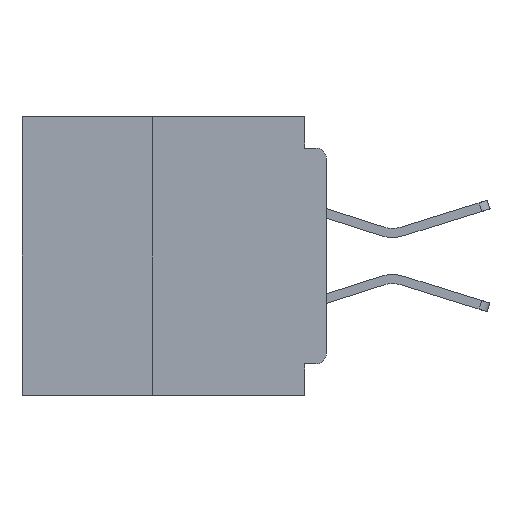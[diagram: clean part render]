
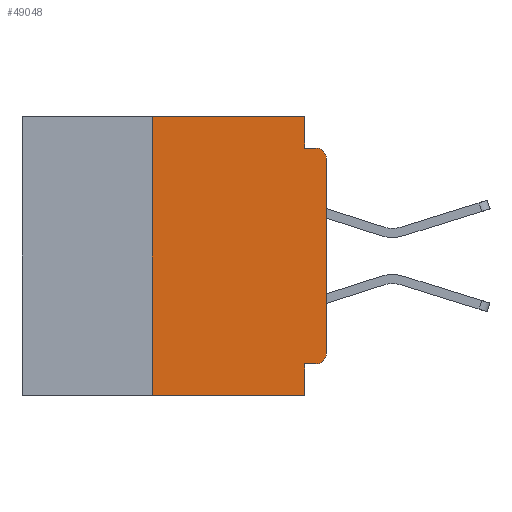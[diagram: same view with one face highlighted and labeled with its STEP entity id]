
A CAD part, left-side view. The second image highlights one B-rep face of the part: STEP entity #49048.
In plain terms, the highlighted planar face has unit normal (-1, 0, 0).
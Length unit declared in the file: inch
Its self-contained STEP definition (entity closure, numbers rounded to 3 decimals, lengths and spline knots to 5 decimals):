
#20 = LINE ( 'NONE', #26239, #21455 ) ;
#35 = EDGE_CURVE ( 'NONE', #26544, #19122, #11716, .T. ) ;
#307 = VECTOR ( 'NONE', #14128, 39.37008 ) ;
#1323 = ORIENTED_EDGE ( 'NONE', *, *, #14427, .F. ) ;
#2789 = CARTESIAN_POINT ( 'NONE',  ( 0., 0., -0.045 ) ) ;
#2907 = EDGE_CURVE ( 'NONE', #47723, #47539, #22066, .T. ) ;
#3143 = DIRECTION ( 'NONE',  ( -1., 0., 0. ) ) ;
#3604 = DIRECTION ( 'NONE',  ( 0., 0., -1. ) ) ;
#3890 = DIRECTION ( 'NONE',  ( 0., 0., -1. ) ) ;
#4039 = VERTEX_POINT ( 'NONE', #25247 ) ;
#4975 = LINE ( 'NONE', #16360, #26354 ) ;
#5308 = ORIENTED_EDGE ( 'NONE', *, *, #29322, .F. ) ;
#5551 = CARTESIAN_POINT ( 'NONE',  ( 0., 0., -0.355 ) ) ;
#8605 = AXIS2_PLACEMENT_3D ( 'NONE', #28709, #3143, #33030 ) ;
#9223 = LINE ( 'NONE', #5551, #20586 ) ;
#9282 = DIRECTION ( 'NONE',  ( 0., 0., 1. ) ) ;
#9868 = DIRECTION ( 'NONE',  ( 0., 1., 0. ) ) ;
#10006 = ORIENTED_EDGE ( 'NONE', *, *, #25366, .T. ) ;
#10900 = CARTESIAN_POINT ( 'NONE',  ( 0., 0.031, 0. ) ) ;
#11251 = FACE_OUTER_BOUND ( 'NONE', #22748, .T. ) ;
#11534 = EDGE_CURVE ( 'NONE', #47723, #33958, #36647, .T. ) ;
#11557 = ORIENTED_EDGE ( 'NONE', *, *, #49314, .F. ) ;
#11716 = LINE ( 'NONE', #20911, #307 ) ;
#12443 = VERTEX_POINT ( 'NONE', #46389 ) ;
#13977 = VECTOR ( 'NONE', #43879, 39.37008 ) ;
#14128 = DIRECTION ( 'NONE',  ( 0., 0., -1. ) ) ;
#14427 = EDGE_CURVE ( 'NONE', #39113, #33958, #4975, .T. ) ;
#14734 = CARTESIAN_POINT ( 'NONE',  ( 0., 0.031, -0.045 ) ) ;
#16360 = CARTESIAN_POINT ( 'NONE',  ( 0., 0.031, -0.4 ) ) ;
#16867 = EDGE_CURVE ( 'NONE', #4039, #47789, #35432, .T. ) ;
#17619 = DIRECTION ( 'NONE',  ( 0., -1., 0. ) ) ;
#19122 = VERTEX_POINT ( 'NONE', #14734 ) ;
#19386 = VECTOR ( 'NONE', #49608, 39.37008 ) ;
#19668 = ORIENTED_EDGE ( 'NONE', *, *, #11534, .T. ) ;
#20367 = ORIENTED_EDGE ( 'NONE', *, *, #16867, .T. ) ;
#20586 = VECTOR ( 'NONE', #9868, 39.37008 ) ;
#20911 = CARTESIAN_POINT ( 'NONE',  ( 0., 0.031, 0. ) ) ;
#20925 = DIRECTION ( 'NONE',  ( -1., 0., 0. ) ) ;
#21347 = CARTESIAN_POINT ( 'NONE',  ( 0., 0.25, 0. ) ) ;
#21455 = VECTOR ( 'NONE', #9282, 39.37008 ) ;
#22066 = LINE ( 'NONE', #30630, #43384 ) ;
#22748 = EDGE_LOOP ( 'NONE', ( #41684, #20367, #5308, #37859, #40615, #23875, #19668, #1323, #11557, #10006 ) ) ;
#23367 = VECTOR ( 'NONE', #17619, 39.37008 ) ;
#23875 = ORIENTED_EDGE ( 'NONE', *, *, #2907, .F. ) ;
#25156 = PLANE ( 'NONE',  #40611 ) ;
#25247 = CARTESIAN_POINT ( 'NONE',  ( 0., 0., -0.06 ) ) ;
#25366 = EDGE_CURVE ( 'NONE', #39850, #12443, #53982, .T. ) ;
#26239 = CARTESIAN_POINT ( 'NONE',  ( 0., 0., 0. ) ) ;
#26354 = VECTOR ( 'NONE', #3604, 39.37008 ) ;
#26544 = VERTEX_POINT ( 'NONE', #10900 ) ;
#28709 = CARTESIAN_POINT ( 'NONE',  ( 0., 0.015, -0.34 ) ) ;
#29322 = EDGE_CURVE ( 'NONE', #19122, #47789, #32064, .T. ) ;
#29481 = DIRECTION ( 'NONE',  ( 1., 0., 0. ) ) ;
#30322 = DIRECTION ( 'NONE',  ( 0., 0., 1. ) ) ;
#30630 = CARTESIAN_POINT ( 'NONE',  ( 0., 0.25, -0.4 ) ) ;
#31050 = CARTESIAN_POINT ( 'NONE',  ( 0., 0.437, -0.4 ) ) ;
#32064 = LINE ( 'NONE', #2789, #19386 ) ;
#33030 = DIRECTION ( 'NONE',  ( 0., 0., -1. ) ) ;
#33958 = VERTEX_POINT ( 'NONE', #41734 ) ;
#35282 = CARTESIAN_POINT ( 'NONE',  ( 0., 0.031, -0.355 ) ) ;
#35314 = CARTESIAN_POINT ( 'NONE',  ( 0., 0.25, -0.4 ) ) ;
#35432 = CIRCLE ( 'NONE', #51142, 0.015 ) ;
#36647 = LINE ( 'NONE', #31050, #13977 ) ;
#37139 = CARTESIAN_POINT ( 'NONE',  ( 0., 0.015, -0.355 ) ) ;
#37859 = ORIENTED_EDGE ( 'NONE', *, *, #35, .F. ) ;
#39113 = VERTEX_POINT ( 'NONE', #35282 ) ;
#39850 = VERTEX_POINT ( 'NONE', #37139 ) ;
#40611 = AXIS2_PLACEMENT_3D ( 'NONE', #54978, #29481, #3890 ) ;
#40615 = ORIENTED_EDGE ( 'NONE', *, *, #45852, .F. ) ;
#41684 = ORIENTED_EDGE ( 'NONE', *, *, #53210, .T. ) ;
#41734 = CARTESIAN_POINT ( 'NONE',  ( 0., 0.031, -0.4 ) ) ;
#43384 = VECTOR ( 'NONE', #30322, 39.37008 ) ;
#43879 = DIRECTION ( 'NONE',  ( 0., -1., 0. ) ) ;
#44717 = LINE ( 'NONE', #47403, #23367 ) ;
#45852 = EDGE_CURVE ( 'NONE', #47539, #26544, #44717, .T. ) ;
#46389 = CARTESIAN_POINT ( 'NONE',  ( 0., 0., -0.34 ) ) ;
#46436 = CARTESIAN_POINT ( 'NONE',  ( 0., 0.015, -0.06 ) ) ;
#47403 = CARTESIAN_POINT ( 'NONE',  ( 0., 0.437, 0. ) ) ;
#47539 = VERTEX_POINT ( 'NONE', #21347 ) ;
#47723 = VERTEX_POINT ( 'NONE', #35314 ) ;
#47789 = VERTEX_POINT ( 'NONE', #52763 ) ;
#49048 = ADVANCED_FACE ( 'NONE', ( #11251 ), #25156, .F. ) ;
#49314 = EDGE_CURVE ( 'NONE', #39850, #39113, #9223, .T. ) ;
#49608 = DIRECTION ( 'NONE',  ( 0., -1., 0. ) ) ;
#50728 = DIRECTION ( 'NONE',  ( 0., 0., -1. ) ) ;
#51142 = AXIS2_PLACEMENT_3D ( 'NONE', #46436, #20925, #50728 ) ;
#52763 = CARTESIAN_POINT ( 'NONE',  ( 0., 0.015, -0.045 ) ) ;
#53210 = EDGE_CURVE ( 'NONE', #12443, #4039, #20, .T. ) ;
#53982 = CIRCLE ( 'NONE', #8605, 0.015 ) ;
#54978 = CARTESIAN_POINT ( 'NONE',  ( 0., 0.437, 0. ) ) ;
